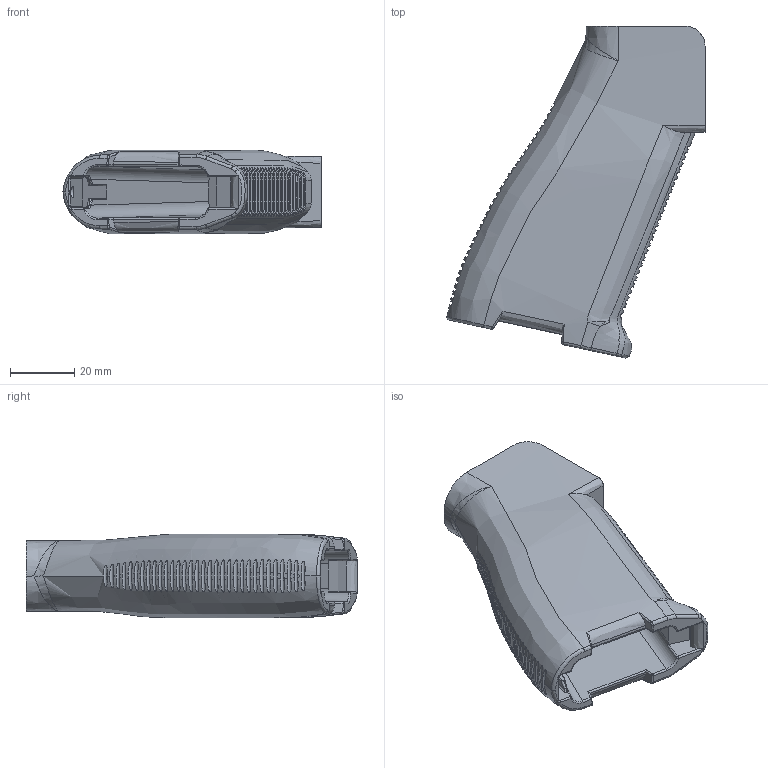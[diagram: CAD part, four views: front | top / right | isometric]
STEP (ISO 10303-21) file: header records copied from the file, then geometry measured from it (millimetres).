
FILE_DESCRIPTION(/* description */ (''),/* implementation_level */ '2;1');
FILE_NAME(/* name */ 'Py2A Get A Grip.step',/* time_stamp */ '2022-07-29T19:17:58-04:00',/* author */ (''),/* organization */ (''),/* preprocessor_version */ 'ST-DEVELOPER v19',/* originating_system */ 'Autodesk Translation Framework v11.7.0.108',/* authorisation */ '');
FILE_SCHEMA (('AUTOMOTIVE_DESIGN { 1 0 10303 214 3 1 1 }'));
Products named in the file (1): AR-15_Grip
Bounding box: 80.23 x 103.17 x 25.98 mm (x, y, z)
Volume: 59875.2 mm3; surface area: 24838.8 mm2
Topology: 1 solids, 1 shells, 357 faces, 1113 edges, 751 vertices
Faces by surface type: bspline 173, cylinder 91, plane 84, sphere 9
Full cylindrical faces by diameter (mm): 3.2 x1, 6.65 x1
Entity records: 37679 total; most frequent: CARTESIAN_POINT 29679, ORIENTED_EDGE 2200, EDGE_CURVE 1100, DIRECTION 872, VERTEX_POINT 753, B_SPLINE_CURVE_WITH_KNOTS 697, EDGE_LOOP 367, FACE_OUTER_BOUND 357
